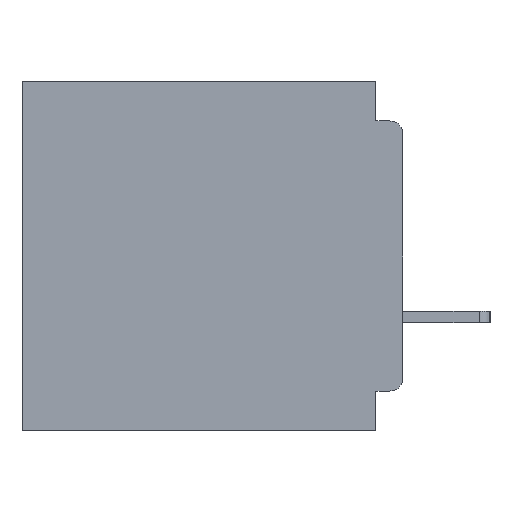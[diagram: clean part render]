
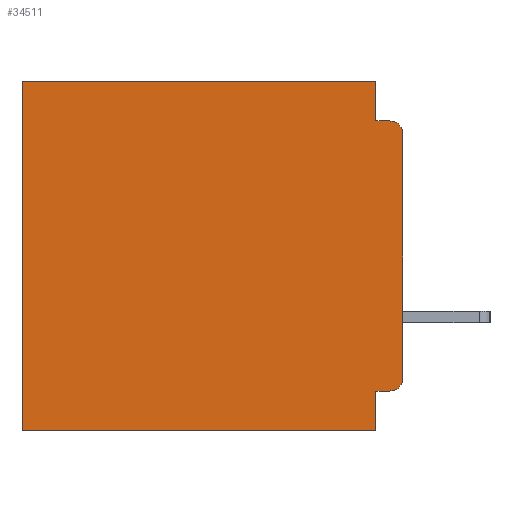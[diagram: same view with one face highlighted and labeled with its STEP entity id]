
A CAD part, left-side view. The second image highlights one B-rep face of the part: STEP entity #34511.
In plain terms, the highlighted planar face has unit normal (-1, 0, 0).
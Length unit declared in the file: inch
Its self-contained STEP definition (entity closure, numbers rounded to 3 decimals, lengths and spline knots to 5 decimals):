
#7 = VERTEX_POINT ( 'NONE', #18447 ) ;
#236 = CARTESIAN_POINT ( 'NONE',  ( 0.3, 0.031, -0.4 ) ) ;
#576 = VERTEX_POINT ( 'NONE', #10653 ) ;
#935 = VECTOR ( 'NONE', #15882, 39.37008 ) ;
#1060 = LINE ( 'NONE', #2411, #29532 ) ;
#1167 = CARTESIAN_POINT ( 'NONE',  ( 0.3, 0.015, -0.34 ) ) ;
#1629 = CARTESIAN_POINT ( 'NONE',  ( 0.3, 0.015, -0.045 ) ) ;
#1781 = LINE ( 'NONE', #3303, #15702 ) ;
#2020 = ORIENTED_EDGE ( 'NONE', *, *, #8421, .F. ) ;
#2159 = VERTEX_POINT ( 'NONE', #1629 ) ;
#2411 = CARTESIAN_POINT ( 'NONE',  ( 0.3, 0.437, -0.4 ) ) ;
#3303 = CARTESIAN_POINT ( 'NONE',  ( 0.3, 0.031, -0.4 ) ) ;
#3435 = EDGE_CURVE ( 'NONE', #11595, #23651, #1060, .T. ) ;
#4027 = DIRECTION ( 'NONE',  ( 0., 0., -1. ) ) ;
#4140 = CARTESIAN_POINT ( 'NONE',  ( 0.3, 0., -0.045 ) ) ;
#4346 = LINE ( 'NONE', #4140, #26297 ) ;
#4448 = LINE ( 'NONE', #16856, #18260 ) ;
#4660 = ORIENTED_EDGE ( 'NONE', *, *, #13484, .T. ) ;
#5997 = EDGE_CURVE ( 'NONE', #16188, #20069, #13294, .T. ) ;
#6106 = DIRECTION ( 'NONE',  ( 0., 0., -1. ) ) ;
#7354 = VERTEX_POINT ( 'NONE', #30809 ) ;
#8176 = EDGE_CURVE ( 'NONE', #7354, #7, #25989, .T. ) ;
#8374 = EDGE_CURVE ( 'NONE', #576, #34296, #4448, .T. ) ;
#8421 = EDGE_CURVE ( 'NONE', #20069, #19407, #1781, .T. ) ;
#9008 = ORIENTED_EDGE ( 'NONE', *, *, #8374, .F. ) ;
#10354 = EDGE_CURVE ( 'NONE', #34296, #2159, #4346, .T. ) ;
#10563 = CIRCLE ( 'NONE', #24802, 0.015 ) ;
#10653 = CARTESIAN_POINT ( 'NONE',  ( 0.3, 0.031, 0. ) ) ;
#11567 = VECTOR ( 'NONE', #21525, 39.37008 ) ;
#11595 = VERTEX_POINT ( 'NONE', #24360 ) ;
#11604 = CARTESIAN_POINT ( 'NONE',  ( 0.3, 0.015, -0.355 ) ) ;
#13082 = LINE ( 'NONE', #18854, #34839 ) ;
#13201 = CARTESIAN_POINT ( 'NONE',  ( 0.3, 0.437, -0.4 ) ) ;
#13237 = CARTESIAN_POINT ( 'NONE',  ( 0.3, 0., -0.4 ) ) ;
#13294 = LINE ( 'NONE', #21491, #11567 ) ;
#13484 = EDGE_CURVE ( 'NONE', #7354, #2159, #31492, .T. ) ;
#14509 = CARTESIAN_POINT ( 'NONE',  ( 0.3, 0.015, -0.06 ) ) ;
#14534 = EDGE_CURVE ( 'NONE', #19407, #23651, #13082, .T. ) ;
#15702 = VECTOR ( 'NONE', #6106, 39.37008 ) ;
#15729 = LINE ( 'NONE', #24010, #935 ) ;
#15882 = DIRECTION ( 'NONE',  ( 0., 1., 0. ) ) ;
#16188 = VERTEX_POINT ( 'NONE', #11604 ) ;
#16208 = CARTESIAN_POINT ( 'NONE',  ( 0.3, 0., -0.4 ) ) ;
#16348 = ORIENTED_EDGE ( 'NONE', *, *, #28808, .T. ) ;
#16856 = CARTESIAN_POINT ( 'NONE',  ( 0.3, 0.031, 0. ) ) ;
#17276 = DIRECTION ( 'NONE',  ( 0., 0., -1. ) ) ;
#17515 = AXIS2_PLACEMENT_3D ( 'NONE', #14509, #33557, #17276 ) ;
#18047 = ORIENTED_EDGE ( 'NONE', *, *, #3435, .T. ) ;
#18260 = VECTOR ( 'NONE', #33144, 39.37008 ) ;
#18447 = CARTESIAN_POINT ( 'NONE',  ( 0.3, 0., -0.34 ) ) ;
#18854 = CARTESIAN_POINT ( 'NONE',  ( 0.3, 0., -0.4 ) ) ;
#18923 = DIRECTION ( 'NONE',  ( 0., 0., -1. ) ) ;
#19108 = AXIS2_PLACEMENT_3D ( 'NONE', #16208, #35224, #18923 ) ;
#19407 = VERTEX_POINT ( 'NONE', #236 ) ;
#20069 = VERTEX_POINT ( 'NONE', #33613 ) ;
#20519 = DIRECTION ( 'NONE',  ( -1., 0., 0. ) ) ;
#20581 = DIRECTION ( 'NONE',  ( 0., 0., -1. ) ) ;
#21113 = FACE_OUTER_BOUND ( 'NONE', #25028, .T. ) ;
#21491 = CARTESIAN_POINT ( 'NONE',  ( 0.3, 0., -0.355 ) ) ;
#21525 = DIRECTION ( 'NONE',  ( 0., 1., 0. ) ) ;
#23651 = VERTEX_POINT ( 'NONE', #13201 ) ;
#24010 = CARTESIAN_POINT ( 'NONE',  ( 0.3, 0., 0. ) ) ;
#24360 = CARTESIAN_POINT ( 'NONE',  ( 0.3, 0.437, 0. ) ) ;
#24802 = AXIS2_PLACEMENT_3D ( 'NONE', #1167, #20519, #4027 ) ;
#25028 = EDGE_LOOP ( 'NONE', ( #32943, #4660, #35490, #9008, #16348, #18047, #34215, #2020, #31299, #32982 ) ) ;
#25989 = LINE ( 'NONE', #13237, #32338 ) ;
#26022 = CARTESIAN_POINT ( 'NONE',  ( 0.3, 0.031, -0.045 ) ) ;
#26297 = VECTOR ( 'NONE', #34184, 39.37008 ) ;
#28808 = EDGE_CURVE ( 'NONE', #576, #11595, #15729, .T. ) ;
#29532 = VECTOR ( 'NONE', #20581, 39.37008 ) ;
#29654 = DIRECTION ( 'NONE',  ( 0., 0., -1. ) ) ;
#30809 = CARTESIAN_POINT ( 'NONE',  ( 0.3, 0., -0.06 ) ) ;
#31299 = ORIENTED_EDGE ( 'NONE', *, *, #5997, .F. ) ;
#31439 = EDGE_CURVE ( 'NONE', #16188, #7, #10563, .T. ) ;
#31492 = CIRCLE ( 'NONE', #17515, 0.015 ) ;
#32338 = VECTOR ( 'NONE', #29654, 39.37008 ) ;
#32506 = PLANE ( 'NONE',  #19108 ) ;
#32943 = ORIENTED_EDGE ( 'NONE', *, *, #8176, .F. ) ;
#32982 = ORIENTED_EDGE ( 'NONE', *, *, #31439, .T. ) ;
#33144 = DIRECTION ( 'NONE',  ( 0., 0., -1. ) ) ;
#33557 = DIRECTION ( 'NONE',  ( -1., 0., 0. ) ) ;
#33613 = CARTESIAN_POINT ( 'NONE',  ( 0.3, 0.031, -0.355 ) ) ;
#34184 = DIRECTION ( 'NONE',  ( 0., -1., 0. ) ) ;
#34215 = ORIENTED_EDGE ( 'NONE', *, *, #14534, .F. ) ;
#34296 = VERTEX_POINT ( 'NONE', #26022 ) ;
#34511 = ADVANCED_FACE ( 'NONE', ( #21113 ), #32506, .F. ) ;
#34839 = VECTOR ( 'NONE', #35138, 39.37008 ) ;
#35138 = DIRECTION ( 'NONE',  ( 0., 1., 0. ) ) ;
#35224 = DIRECTION ( 'NONE',  ( 1., 0., 0. ) ) ;
#35490 = ORIENTED_EDGE ( 'NONE', *, *, #10354, .F. ) ;
